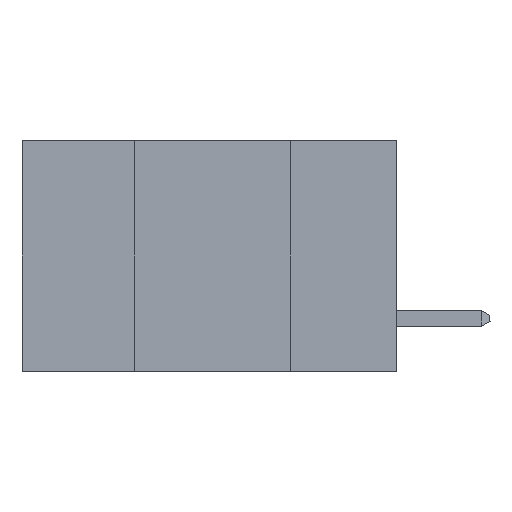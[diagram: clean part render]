
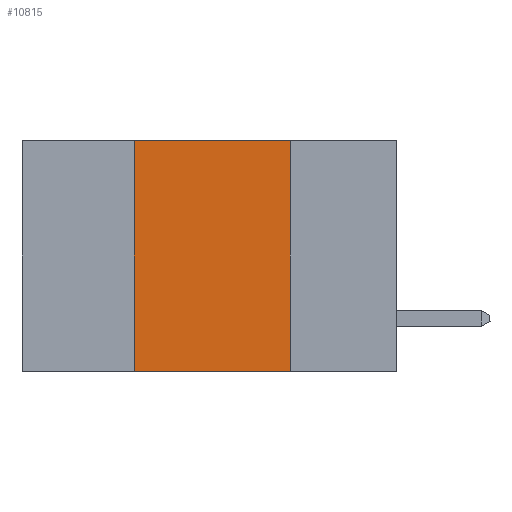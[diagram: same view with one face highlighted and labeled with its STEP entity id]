
A CAD part, left-side view. The second image highlights one B-rep face of the part: STEP entity #10815.
In plain terms, the highlighted planar face has unit normal (-1, 0, 0).
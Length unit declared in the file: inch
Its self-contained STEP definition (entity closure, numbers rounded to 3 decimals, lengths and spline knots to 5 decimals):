
#1573 = CARTESIAN_POINT ( 'NONE',  ( 0., 0.6, 0. ) ) ;
#2218 = VERTEX_POINT ( 'NONE', #3840 ) ;
#3746 = DIRECTION ( 'NONE',  ( 0., 0., -1. ) ) ;
#3840 = CARTESIAN_POINT ( 'NONE',  ( 0., 0.42, -0.37 ) ) ;
#4029 = EDGE_LOOP ( 'NONE', ( #6365, #24512, #14695, #9718 ) ) ;
#5136 = LINE ( 'NONE', #26784, #21113 ) ;
#5916 = EDGE_CURVE ( 'NONE', #9482, #24061, #6694, .T. ) ;
#6311 = VERTEX_POINT ( 'NONE', #20700 ) ;
#6365 = ORIENTED_EDGE ( 'NONE', *, *, #17797, .F. ) ;
#6694 = LINE ( 'NONE', #11275, #22582 ) ;
#7407 = FACE_OUTER_BOUND ( 'NONE', #4029, .T. ) ;
#8267 = CARTESIAN_POINT ( 'NONE',  ( 0., 0.17, 0. ) ) ;
#8581 = DIRECTION ( 'NONE',  ( 0., 0., 1. ) ) ;
#9482 = VERTEX_POINT ( 'NONE', #25860 ) ;
#9718 = ORIENTED_EDGE ( 'NONE', *, *, #15066, .T. ) ;
#10815 = ADVANCED_FACE ( 'NONE', ( #7407 ), #24488, .F. ) ;
#10984 = VECTOR ( 'NONE', #14586, 39.37008 ) ;
#11275 = CARTESIAN_POINT ( 'NONE',  ( 0., 0.6, 0. ) ) ;
#13375 = DIRECTION ( 'NONE',  ( 0., -1., 0. ) ) ;
#14576 = LINE ( 'NONE', #8267, #10984 ) ;
#14586 = DIRECTION ( 'NONE',  ( 0., 0., -1. ) ) ;
#14695 = ORIENTED_EDGE ( 'NONE', *, *, #16443, .F. ) ;
#15066 = EDGE_CURVE ( 'NONE', #2218, #6311, #5136, .T. ) ;
#16375 = DIRECTION ( 'NONE',  ( 1., 0., 0. ) ) ;
#16443 = EDGE_CURVE ( 'NONE', #2218, #9482, #17852, .T. ) ;
#16655 = DIRECTION ( 'NONE',  ( 0., -1., 0. ) ) ;
#17201 = AXIS2_PLACEMENT_3D ( 'NONE', #1573, #16375, #3746 ) ;
#17204 = VECTOR ( 'NONE', #8581, 39.37008 ) ;
#17797 = EDGE_CURVE ( 'NONE', #24061, #6311, #14576, .T. ) ;
#17852 = LINE ( 'NONE', #18897, #17204 ) ;
#18519 = CARTESIAN_POINT ( 'NONE',  ( 0., 0.17, 0. ) ) ;
#18897 = CARTESIAN_POINT ( 'NONE',  ( 0., 0.42, 0. ) ) ;
#20700 = CARTESIAN_POINT ( 'NONE',  ( 0., 0.17, -0.37 ) ) ;
#21113 = VECTOR ( 'NONE', #16655, 39.37008 ) ;
#22582 = VECTOR ( 'NONE', #13375, 39.37008 ) ;
#24061 = VERTEX_POINT ( 'NONE', #18519 ) ;
#24488 = PLANE ( 'NONE',  #17201 ) ;
#24512 = ORIENTED_EDGE ( 'NONE', *, *, #5916, .F. ) ;
#25860 = CARTESIAN_POINT ( 'NONE',  ( 0., 0.42, 0. ) ) ;
#26784 = CARTESIAN_POINT ( 'NONE',  ( 0., 0.6, -0.37 ) ) ;
